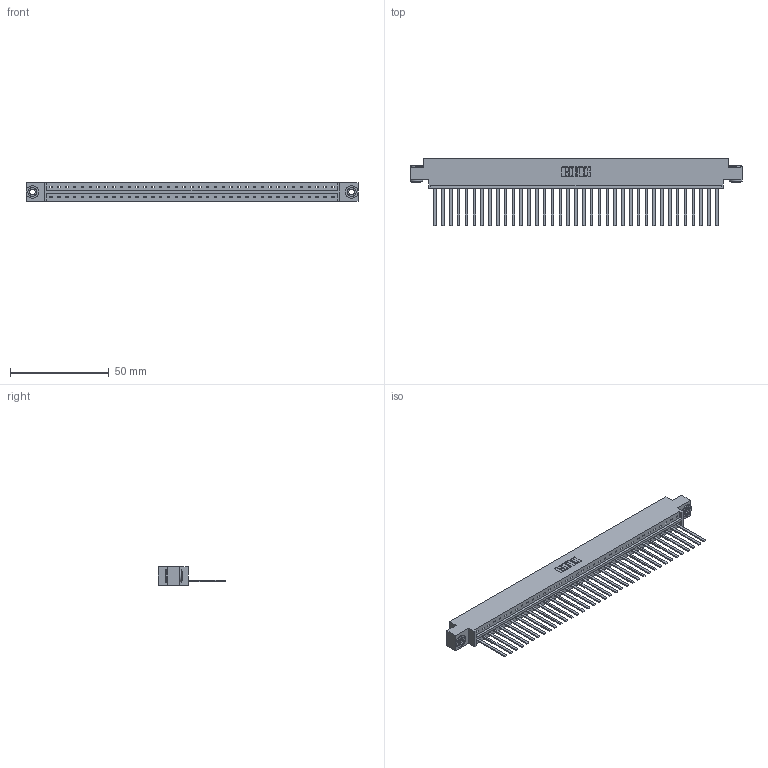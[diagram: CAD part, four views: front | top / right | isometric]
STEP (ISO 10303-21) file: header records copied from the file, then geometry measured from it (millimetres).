
FILE_DESCRIPTION (( 'STEP AP203' ), '1' );
FILE_NAME ('833-037-544-603.STEP', '2020-06-03T05:39:48', ( '' ), ( '' ), 'SwSTEP 2.0', 'SolidWorks 2020', '' );
FILE_SCHEMA (( 'CONFIG_CONTROL_DESIGN' ));
Length unit declared in the file: inch
Products named in the file (4): 833 Part_Offset - .156 Dia - TH; 345-292-001_345-293-144; 345-250-002_345-250-002-102; 833-037-544-603
Assembly tree (40 placements, depth 2):
  833-037-544-603
    833 Part_Offset - .156 Dia - TH
    345-292-001_345-293-144  x37
    345-250-002_345-250-002-102  x2
Bounding box: 168.15 x 34.3 x 9.4 mm (x, y, z)
Volume: 17097.5 mm3; surface area: 20285.5 mm2
Topology: 40 solids, 40 shells, 2080 faces, 6245 edges, 4110 vertices
Faces by surface type: plane 1490, cylinder 582, cone 8
Entity records: 23864 total; most frequent: CARTESIAN_POINT 4096, ORIENTED_EDGE 4062, DIRECTION 3495, EDGE_CURVE 2031, VECTOR 1883, LINE 1883, VERTEX_POINT 1350, AXIS2_PLACEMENT_3D 806
